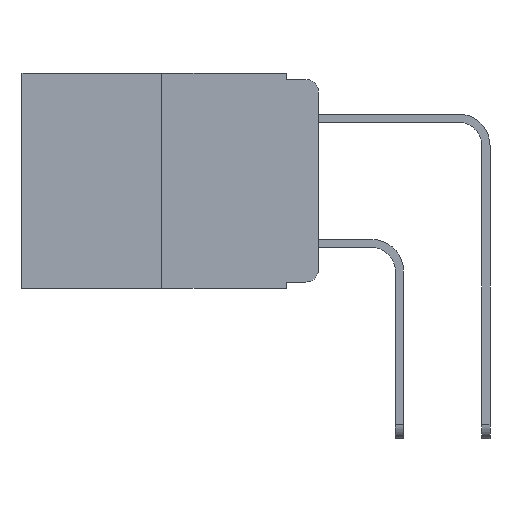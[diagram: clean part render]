
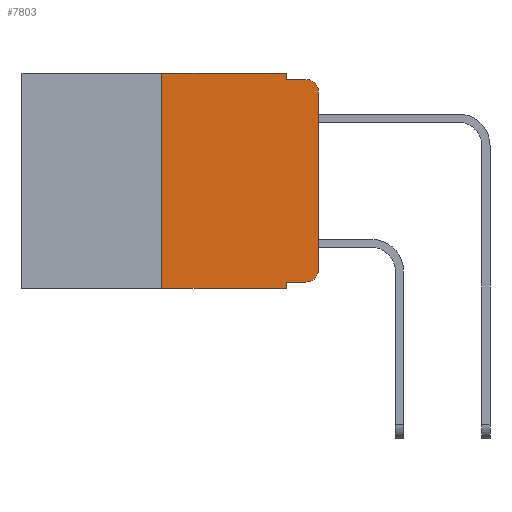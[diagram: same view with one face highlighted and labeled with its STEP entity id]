
A CAD part, left-side view. The second image highlights one B-rep face of the part: STEP entity #7803.
In plain terms, the highlighted planar face has unit normal (-1, 0, 0).
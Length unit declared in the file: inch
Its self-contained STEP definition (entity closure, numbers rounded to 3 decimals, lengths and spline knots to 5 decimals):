
#118 = LINE ( 'NONE', #13647, #490 ) ;
#490 = VECTOR ( 'NONE', #7564, 39.37008 ) ;
#627 = LINE ( 'NONE', #8411, #3669 ) ;
#660 = DIRECTION ( 'NONE',  ( 1., 0., 0. ) ) ;
#666 = VERTEX_POINT ( 'NONE', #10935 ) ;
#731 = DIRECTION ( 'NONE',  ( -1., 0., 0. ) ) ;
#938 = DIRECTION ( 'NONE',  ( 0., 0., 1. ) ) ;
#1011 = ORIENTED_EDGE ( 'NONE', *, *, #3684, .T. ) ;
#1220 = CARTESIAN_POINT ( 'NONE',  ( 0., 0.051, -0.333 ) ) ;
#1547 = ORIENTED_EDGE ( 'NONE', *, *, #8126, .T. ) ;
#1769 = VECTOR ( 'NONE', #8863, 39.37008 ) ;
#1874 = DIRECTION ( 'NONE',  ( 0., 0., -1. ) ) ;
#1973 = CARTESIAN_POINT ( 'NONE',  ( 0., 0.051, -0.01 ) ) ;
#2135 = LINE ( 'NONE', #1220, #1769 ) ;
#2222 = VECTOR ( 'NONE', #9659, 39.37008 ) ;
#2714 = VERTEX_POINT ( 'NONE', #5060 ) ;
#2831 = VECTOR ( 'NONE', #10770, 39.37008 ) ;
#2967 = ORIENTED_EDGE ( 'NONE', *, *, #8222, .F. ) ;
#3019 = EDGE_CURVE ( 'NONE', #8050, #7470, #5965, .T. ) ;
#3183 = DIRECTION ( 'NONE',  ( 0., -1., 0. ) ) ;
#3357 = CARTESIAN_POINT ( 'NONE',  ( 0., 0.473, -0.343 ) ) ;
#3669 = VECTOR ( 'NONE', #1874, 39.37008 ) ;
#3684 = EDGE_CURVE ( 'NONE', #666, #5544, #9240, .T. ) ;
#3768 = EDGE_CURVE ( 'NONE', #4499, #8050, #2135, .T. ) ;
#3962 = CARTESIAN_POINT ( 'NONE',  ( 0., 0.02, -0.333 ) ) ;
#4432 = DIRECTION ( 'NONE',  ( -1., 0., 0. ) ) ;
#4439 = DIRECTION ( 'NONE',  ( 0., -1., 0. ) ) ;
#4499 = VERTEX_POINT ( 'NONE', #8973 ) ;
#4637 = VECTOR ( 'NONE', #4439, 39.37008 ) ;
#4661 = CARTESIAN_POINT ( 'NONE',  ( 0., 0.051, -0.343 ) ) ;
#5060 = CARTESIAN_POINT ( 'NONE',  ( 0., 0.051, 0. ) ) ;
#5236 = EDGE_CURVE ( 'NONE', #4499, #5544, #627, .T. ) ;
#5296 = VERTEX_POINT ( 'NONE', #1973 ) ;
#5544 = VERTEX_POINT ( 'NONE', #4661 ) ;
#5563 = CARTESIAN_POINT ( 'NONE',  ( 0., 0.051, -0.01 ) ) ;
#5617 = CARTESIAN_POINT ( 'NONE',  ( 0., 0.25, 0. ) ) ;
#5965 = CIRCLE ( 'NONE', #11451, 0.02 ) ;
#5974 = EDGE_CURVE ( 'NONE', #666, #9580, #8860, .T. ) ;
#6242 = CARTESIAN_POINT ( 'NONE',  ( 0., 0.02, -0.01 ) ) ;
#6254 = CARTESIAN_POINT ( 'NONE',  ( 0., 0.473, 0. ) ) ;
#6518 = CARTESIAN_POINT ( 'NONE',  ( 0., 0.051, 0. ) ) ;
#6585 = ORIENTED_EDGE ( 'NONE', *, *, #5974, .F. ) ;
#6706 = EDGE_CURVE ( 'NONE', #2714, #5296, #10734, .T. ) ;
#7088 = ORIENTED_EDGE ( 'NONE', *, *, #3019, .T. ) ;
#7354 = VERTEX_POINT ( 'NONE', #9641 ) ;
#7394 = CARTESIAN_POINT ( 'NONE',  ( 0., 0.02, -0.03 ) ) ;
#7422 = EDGE_CURVE ( 'NONE', #5296, #12952, #10236, .T. ) ;
#7470 = VERTEX_POINT ( 'NONE', #8836 ) ;
#7564 = DIRECTION ( 'NONE',  ( 0., 0., 1. ) ) ;
#7803 = ADVANCED_FACE ( 'NONE', ( #7838 ), #13436, .F. ) ;
#7838 = FACE_OUTER_BOUND ( 'NONE', #11728, .T. ) ;
#7925 = ORIENTED_EDGE ( 'NONE', *, *, #3768, .T. ) ;
#8050 = VERTEX_POINT ( 'NONE', #3962 ) ;
#8087 = ORIENTED_EDGE ( 'NONE', *, *, #6706, .F. ) ;
#8126 = EDGE_CURVE ( 'NONE', #7354, #12952, #12122, .T. ) ;
#8222 = EDGE_CURVE ( 'NONE', #9580, #2714, #8783, .T. ) ;
#8376 = DIRECTION ( 'NONE',  ( 0., 0., -1. ) ) ;
#8411 = CARTESIAN_POINT ( 'NONE',  ( 0., 0.051, 0. ) ) ;
#8433 = DIRECTION ( 'NONE',  ( 0., 0., -1. ) ) ;
#8783 = LINE ( 'NONE', #10573, #10848 ) ;
#8806 = EDGE_CURVE ( 'NONE', #7470, #7354, #118, .T. ) ;
#8836 = CARTESIAN_POINT ( 'NONE',  ( 0., 0., -0.313 ) ) ;
#8860 = LINE ( 'NONE', #11641, #10920 ) ;
#8863 = DIRECTION ( 'NONE',  ( 0., -1., 0. ) ) ;
#8973 = CARTESIAN_POINT ( 'NONE',  ( 0., 0.051, -0.333 ) ) ;
#9240 = LINE ( 'NONE', #3357, #2831 ) ;
#9376 = AXIS2_PLACEMENT_3D ( 'NONE', #6254, #660, #8376 ) ;
#9580 = VERTEX_POINT ( 'NONE', #5617 ) ;
#9641 = CARTESIAN_POINT ( 'NONE',  ( 0., 0., -0.03 ) ) ;
#9659 = DIRECTION ( 'NONE',  ( 0., 0., -1. ) ) ;
#9825 = ORIENTED_EDGE ( 'NONE', *, *, #8806, .T. ) ;
#10236 = LINE ( 'NONE', #5563, #4637 ) ;
#10483 = AXIS2_PLACEMENT_3D ( 'NONE', #7394, #731, #8433 ) ;
#10573 = CARTESIAN_POINT ( 'NONE',  ( 0., 0.473, 0. ) ) ;
#10734 = LINE ( 'NONE', #6518, #2222 ) ;
#10741 = CARTESIAN_POINT ( 'NONE',  ( 0., 0.02, -0.313 ) ) ;
#10770 = DIRECTION ( 'NONE',  ( 0., -1., 0. ) ) ;
#10848 = VECTOR ( 'NONE', #3183, 39.37008 ) ;
#10920 = VECTOR ( 'NONE', #938, 39.37008 ) ;
#10935 = CARTESIAN_POINT ( 'NONE',  ( 0., 0.25, -0.343 ) ) ;
#11451 = AXIS2_PLACEMENT_3D ( 'NONE', #10741, #4432, #11767 ) ;
#11641 = CARTESIAN_POINT ( 'NONE',  ( 0., 0.25, 0. ) ) ;
#11728 = EDGE_LOOP ( 'NONE', ( #9825, #1547, #12867, #8087, #2967, #6585, #1011, #12369, #7925, #7088 ) ) ;
#11767 = DIRECTION ( 'NONE',  ( 0., 0., -1. ) ) ;
#12122 = CIRCLE ( 'NONE', #10483, 0.02 ) ;
#12369 = ORIENTED_EDGE ( 'NONE', *, *, #5236, .F. ) ;
#12867 = ORIENTED_EDGE ( 'NONE', *, *, #7422, .F. ) ;
#12952 = VERTEX_POINT ( 'NONE', #6242 ) ;
#13436 = PLANE ( 'NONE',  #9376 ) ;
#13647 = CARTESIAN_POINT ( 'NONE',  ( 0., 0., 0. ) ) ;
